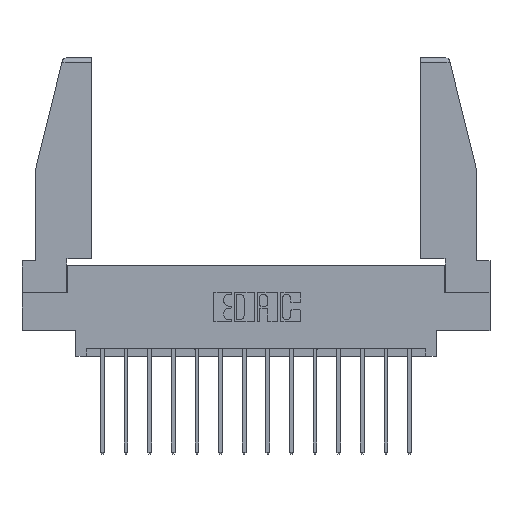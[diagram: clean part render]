
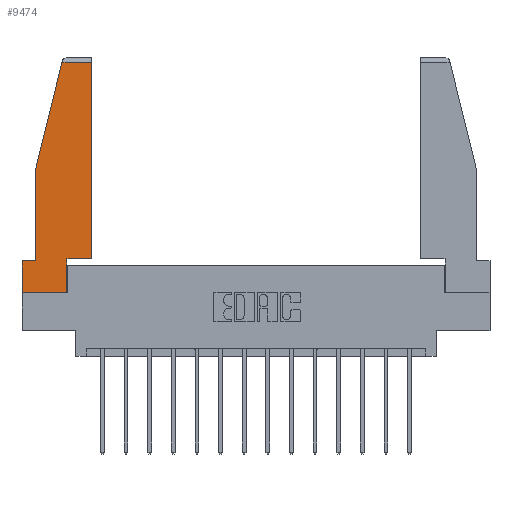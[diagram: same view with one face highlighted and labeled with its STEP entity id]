
A CAD part, top view. The second image highlights one B-rep face of the part: STEP entity #9474.
In plain terms, the highlighted planar face has unit normal (0, 0, 1).
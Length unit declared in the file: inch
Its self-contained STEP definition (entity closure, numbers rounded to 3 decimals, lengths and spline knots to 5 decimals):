
#132 = EDGE_CURVE ( 'NONE', #2194, #6452, #16361, .T. ) ;
#407 = CARTESIAN_POINT ( 'NONE',  ( 0.297, 0., 0. ) ) ;
#463 = CARTESIAN_POINT ( 'NONE',  ( 0., 0.21, 0. ) ) ;
#504 = CARTESIAN_POINT ( 'NONE',  ( 0.297, 0., 0. ) ) ;
#815 = VERTEX_POINT ( 'NONE', #504 ) ;
#824 = DIRECTION ( 'NONE',  ( -1., 0., 0. ) ) ;
#1191 = EDGE_CURVE ( 'NONE', #6452, #815, #4964, .T. ) ;
#2192 = ORIENTED_EDGE ( 'NONE', *, *, #1191, .T. ) ;
#2194 = VERTEX_POINT ( 'NONE', #15039 ) ;
#2281 = ORIENTED_EDGE ( 'NONE', *, *, #132, .T. ) ;
#2878 = DIRECTION ( 'NONE',  ( 0., 1., 0. ) ) ;
#3105 = CARTESIAN_POINT ( 'NONE',  ( 0.086, 0.8, 0. ) ) ;
#3118 = CARTESIAN_POINT ( 'NONE',  ( 0.297, 0.223, 0. ) ) ;
#3174 = ORIENTED_EDGE ( 'NONE', *, *, #14005, .T. ) ;
#3619 = VECTOR ( 'NONE', #15283, 39.37008 ) ;
#3798 = EDGE_CURVE ( 'NONE', #16898, #9835, #8554, .T. ) ;
#4790 = DIRECTION ( 'NONE',  ( 0., 0., 1. ) ) ;
#4964 = LINE ( 'NONE', #13417, #14467 ) ;
#5200 = ORIENTED_EDGE ( 'NONE', *, *, #14606, .T. ) ;
#5225 = VECTOR ( 'NONE', #8144, 39.37008 ) ;
#5244 = EDGE_CURVE ( 'NONE', #8630, #16042, #7688, .T. ) ;
#5414 = VECTOR ( 'NONE', #14923, 39.37008 ) ;
#5439 = VECTOR ( 'NONE', #15393, 39.37008 ) ;
#5471 = LINE ( 'NONE', #5825, #14966 ) ;
#5825 = CARTESIAN_POINT ( 'NONE',  ( 0., 0.21, 0. ) ) ;
#5871 = CARTESIAN_POINT ( 'NONE',  ( 0.297, 0.223, 0. ) ) ;
#6157 = CARTESIAN_POINT ( 'NONE',  ( 0.461, 0.223, 0. ) ) ;
#6452 = VERTEX_POINT ( 'NONE', #14888 ) ;
#6904 = ORIENTED_EDGE ( 'NONE', *, *, #8647, .T. ) ;
#6945 = AXIS2_PLACEMENT_3D ( 'NONE', #16618, #4790, #14022 ) ;
#7524 = LINE ( 'NONE', #5871, #3619 ) ;
#7688 = LINE ( 'NONE', #11948, #5225 ) ;
#7713 = VECTOR ( 'NONE', #2878, 39.37008 ) ;
#7863 = EDGE_CURVE ( 'NONE', #9003, #8313, #7524, .T. ) ;
#7888 = FACE_OUTER_BOUND ( 'NONE', #16986, .T. ) ;
#8144 = DIRECTION ( 'NONE',  ( -1., 0., 0. ) ) ;
#8309 = DIRECTION ( 'NONE',  ( -0.239, -0.971, 0. ) ) ;
#8313 = VERTEX_POINT ( 'NONE', #13806 ) ;
#8338 = CARTESIAN_POINT ( 'NONE',  ( 0.086, 0.21, 0. ) ) ;
#8554 = LINE ( 'NONE', #14840, #16842 ) ;
#8630 = VERTEX_POINT ( 'NONE', #13458 ) ;
#8633 = ORIENTED_EDGE ( 'NONE', *, *, #16857, .T. ) ;
#8647 = EDGE_CURVE ( 'NONE', #815, #9003, #13505, .T. ) ;
#9003 = VERTEX_POINT ( 'NONE', #3118 ) ;
#9154 = ORIENTED_EDGE ( 'NONE', *, *, #7863, .T. ) ;
#9474 = ADVANCED_FACE ( 'NONE', ( #7888 ), #13511, .T. ) ;
#9835 = VERTEX_POINT ( 'NONE', #8338 ) ;
#10641 = CARTESIAN_POINT ( 'NONE',  ( 0.271, 1.55, 0. ) ) ;
#10933 = DIRECTION ( 'NONE',  ( 0., -1., 0. ) ) ;
#11422 = ORIENTED_EDGE ( 'NONE', *, *, #5244, .T. ) ;
#11948 = CARTESIAN_POINT ( 'NONE',  ( 0., 1.52, 0. ) ) ;
#11992 = LINE ( 'NONE', #10641, #15275 ) ;
#12024 = DIRECTION ( 'NONE',  ( 1., 0., 0. ) ) ;
#12723 = ORIENTED_EDGE ( 'NONE', *, *, #3798, .T. ) ;
#13417 = CARTESIAN_POINT ( 'NONE',  ( 0., 0., 0. ) ) ;
#13458 = CARTESIAN_POINT ( 'NONE',  ( 0.461, 1.52, 0. ) ) ;
#13505 = LINE ( 'NONE', #407, #7713 ) ;
#13511 = PLANE ( 'NONE',  #6945 ) ;
#13806 = CARTESIAN_POINT ( 'NONE',  ( 0.461, 0.223, 0. ) ) ;
#14005 = EDGE_CURVE ( 'NONE', #9835, #2194, #5471, .T. ) ;
#14022 = DIRECTION ( 'NONE',  ( 1., 0., 0. ) ) ;
#14128 = LINE ( 'NONE', #6157, #5439 ) ;
#14467 = VECTOR ( 'NONE', #12024, 39.37008 ) ;
#14606 = EDGE_CURVE ( 'NONE', #8313, #8630, #14128, .T. ) ;
#14840 = CARTESIAN_POINT ( 'NONE',  ( 0.086, 0.8, 0. ) ) ;
#14888 = CARTESIAN_POINT ( 'NONE',  ( 0., 0., 0. ) ) ;
#14923 = DIRECTION ( 'NONE',  ( 0., -1., 0. ) ) ;
#14966 = VECTOR ( 'NONE', #824, 39.37008 ) ;
#15039 = CARTESIAN_POINT ( 'NONE',  ( 0., 0.21, 0. ) ) ;
#15275 = VECTOR ( 'NONE', #8309, 39.37008 ) ;
#15283 = DIRECTION ( 'NONE',  ( 1., 0., 0. ) ) ;
#15393 = DIRECTION ( 'NONE',  ( 0., 1., 0. ) ) ;
#15735 = CARTESIAN_POINT ( 'NONE',  ( 0.2636, 1.52, 0. ) ) ;
#16042 = VERTEX_POINT ( 'NONE', #15735 ) ;
#16361 = LINE ( 'NONE', #463, #5414 ) ;
#16618 = CARTESIAN_POINT ( 'NONE',  ( 0., 0., 0. ) ) ;
#16842 = VECTOR ( 'NONE', #10933, 39.37008 ) ;
#16857 = EDGE_CURVE ( 'NONE', #16042, #16898, #11992, .T. ) ;
#16898 = VERTEX_POINT ( 'NONE', #3105 ) ;
#16986 = EDGE_LOOP ( 'NONE', ( #5200, #11422, #8633, #12723, #3174, #2281, #2192, #6904, #9154 ) ) ;
